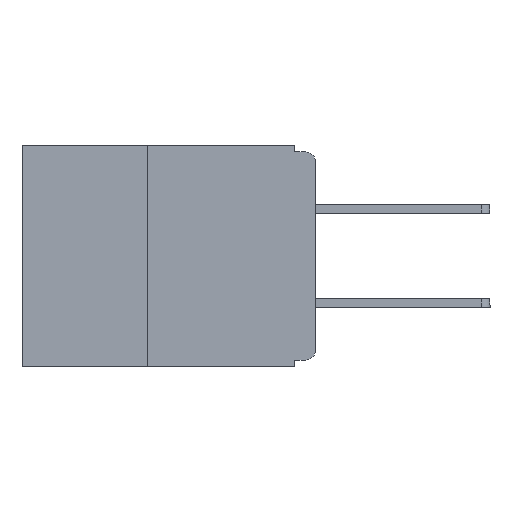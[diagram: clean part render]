
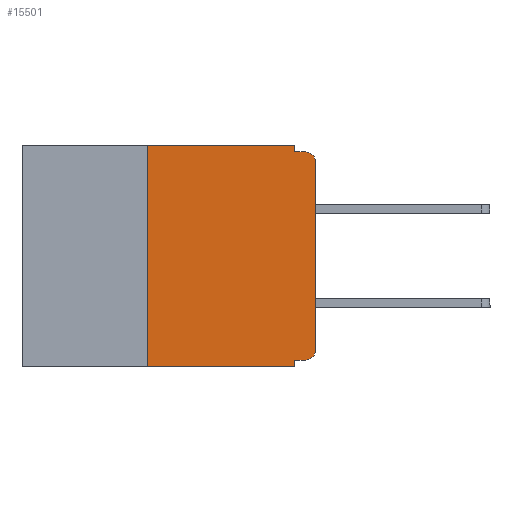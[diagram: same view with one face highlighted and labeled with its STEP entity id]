
A CAD part, left-side view. The second image highlights one B-rep face of the part: STEP entity #15501.
In plain terms, the highlighted planar face has unit normal (-1, 0, 0).
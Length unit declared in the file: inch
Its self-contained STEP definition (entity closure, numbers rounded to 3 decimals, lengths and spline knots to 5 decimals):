
#93 = DIRECTION ( 'NONE',  ( 0., 0., 1. ) ) ;
#161 = DIRECTION ( 'NONE',  ( 0., 0., -1. ) ) ;
#200 = EDGE_CURVE ( 'NONE', #10497, #10987, #3609, .T. ) ;
#527 = ORIENTED_EDGE ( 'NONE', *, *, #200, .T. ) ;
#879 = CARTESIAN_POINT ( 'NONE',  ( 0., 0., -0.025 ) ) ;
#891 = EDGE_CURVE ( 'NONE', #6272, #3194, #23854, .T. ) ;
#1140 = VECTOR ( 'NONE', #13834, 39.37008 ) ;
#1206 = CARTESIAN_POINT ( 'NONE',  ( 0., 0., -0.305 ) ) ;
#1431 = VECTOR ( 'NONE', #21954, 39.37008 ) ;
#2055 = LINE ( 'NONE', #20069, #1431 ) ;
#2853 = VECTOR ( 'NONE', #23637, 39.37008 ) ;
#2869 = EDGE_CURVE ( 'NONE', #10497, #3368, #5034, .T. ) ;
#3194 = VERTEX_POINT ( 'NONE', #1206 ) ;
#3368 = VERTEX_POINT ( 'NONE', #19367 ) ;
#3384 = CARTESIAN_POINT ( 'NONE',  ( 0., 0.437, 0. ) ) ;
#3609 = LINE ( 'NONE', #6363, #23599 ) ;
#3759 = CARTESIAN_POINT ( 'NONE',  ( 0., 0.015, -0.305 ) ) ;
#3777 = VECTOR ( 'NONE', #93, 39.37008 ) ;
#3789 = LINE ( 'NONE', #12873, #18228 ) ;
#4226 = EDGE_CURVE ( 'NONE', #16922, #5382, #19098, .T. ) ;
#4270 = ORIENTED_EDGE ( 'NONE', *, *, #4414, .T. ) ;
#4317 = CARTESIAN_POINT ( 'NONE',  ( 0., 0.015, -0.025 ) ) ;
#4382 = VERTEX_POINT ( 'NONE', #879 ) ;
#4414 = EDGE_CURVE ( 'NONE', #3194, #4382, #3789, .T. ) ;
#5034 = LINE ( 'NONE', #8023, #3777 ) ;
#5382 = VERTEX_POINT ( 'NONE', #17486 ) ;
#5412 = DIRECTION ( 'NONE',  ( 0., -1., 0. ) ) ;
#5519 = ORIENTED_EDGE ( 'NONE', *, *, #19299, .F. ) ;
#5789 = VERTEX_POINT ( 'NONE', #6848 ) ;
#5913 = CARTESIAN_POINT ( 'NONE',  ( 0., 0.031, -0.33 ) ) ;
#6272 = VERTEX_POINT ( 'NONE', #6315 ) ;
#6315 = CARTESIAN_POINT ( 'NONE',  ( 0., 0.015, -0.32 ) ) ;
#6341 = DIRECTION ( 'NONE',  ( 0., 0., -1. ) ) ;
#6363 = CARTESIAN_POINT ( 'NONE',  ( 0., 0.437, -0.33 ) ) ;
#6452 = LINE ( 'NONE', #5913, #1140 ) ;
#6473 = ORIENTED_EDGE ( 'NONE', *, *, #19109, .F. ) ;
#6848 = CARTESIAN_POINT ( 'NONE',  ( 0., 0.031, -0.32 ) ) ;
#7182 = CARTESIAN_POINT ( 'NONE',  ( 0., 0., -0.32 ) ) ;
#7573 = EDGE_CURVE ( 'NONE', #4382, #18886, #15102, .T. ) ;
#7706 = ORIENTED_EDGE ( 'NONE', *, *, #891, .T. ) ;
#7726 = AXIS2_PLACEMENT_3D ( 'NONE', #15925, #12072, #161 ) ;
#7989 = DIRECTION ( 'NONE',  ( 0., -1., 0. ) ) ;
#8023 = CARTESIAN_POINT ( 'NONE',  ( 0., 0.25, -0.33 ) ) ;
#10107 = PLANE ( 'NONE',  #7726 ) ;
#10197 = ORIENTED_EDGE ( 'NONE', *, *, #7573, .T. ) ;
#10256 = EDGE_CURVE ( 'NONE', #6272, #5789, #22152, .T. ) ;
#10322 = CARTESIAN_POINT ( 'NONE',  ( 0., 0.031, 0. ) ) ;
#10497 = VERTEX_POINT ( 'NONE', #11944 ) ;
#10820 = AXIS2_PLACEMENT_3D ( 'NONE', #3759, #22332, #20162 ) ;
#10915 = DIRECTION ( 'NONE',  ( 0., 0., 1. ) ) ;
#10987 = VERTEX_POINT ( 'NONE', #17690 ) ;
#11100 = DIRECTION ( 'NONE',  ( 0., 1., 0. ) ) ;
#11944 = CARTESIAN_POINT ( 'NONE',  ( 0., 0.25, -0.33 ) ) ;
#12041 = ORIENTED_EDGE ( 'NONE', *, *, #17870, .F. ) ;
#12072 = DIRECTION ( 'NONE',  ( 1., 0., 0. ) ) ;
#12873 = CARTESIAN_POINT ( 'NONE',  ( 0., 0., 0. ) ) ;
#13834 = DIRECTION ( 'NONE',  ( 0., 0., -1. ) ) ;
#15102 = CIRCLE ( 'NONE', #15833, 0.015 ) ;
#15501 = ADVANCED_FACE ( 'NONE', ( #20167 ), #10107, .F. ) ;
#15714 = EDGE_LOOP ( 'NONE', ( #4270, #10197, #5519, #16607, #12041, #24472, #527, #6473, #16913, #7706 ) ) ;
#15833 = AXIS2_PLACEMENT_3D ( 'NONE', #4317, #18046, #6341 ) ;
#15925 = CARTESIAN_POINT ( 'NONE',  ( 0., 0.437, 0. ) ) ;
#16607 = ORIENTED_EDGE ( 'NONE', *, *, #4226, .F. ) ;
#16913 = ORIENTED_EDGE ( 'NONE', *, *, #10256, .F. ) ;
#16922 = VERTEX_POINT ( 'NONE', #22348 ) ;
#16960 = VECTOR ( 'NONE', #5412, 39.37008 ) ;
#17486 = CARTESIAN_POINT ( 'NONE',  ( 0., 0.031, -0.01 ) ) ;
#17690 = CARTESIAN_POINT ( 'NONE',  ( 0., 0.031, -0.33 ) ) ;
#17870 = EDGE_CURVE ( 'NONE', #3368, #16922, #21942, .T. ) ;
#18046 = DIRECTION ( 'NONE',  ( -1., 0., 0. ) ) ;
#18228 = VECTOR ( 'NONE', #10915, 39.37008 ) ;
#18862 = CARTESIAN_POINT ( 'NONE',  ( 0., 0.015, -0.01 ) ) ;
#18886 = VERTEX_POINT ( 'NONE', #18862 ) ;
#19098 = LINE ( 'NONE', #10322, #2853 ) ;
#19109 = EDGE_CURVE ( 'NONE', #5789, #10987, #6452, .T. ) ;
#19299 = EDGE_CURVE ( 'NONE', #5382, #18886, #2055, .T. ) ;
#19367 = CARTESIAN_POINT ( 'NONE',  ( 0., 0.25, 0. ) ) ;
#20069 = CARTESIAN_POINT ( 'NONE',  ( 0., 0., -0.01 ) ) ;
#20162 = DIRECTION ( 'NONE',  ( 0., 0., -1. ) ) ;
#20167 = FACE_OUTER_BOUND ( 'NONE', #15714, .T. ) ;
#21580 = VECTOR ( 'NONE', #11100, 39.37008 ) ;
#21942 = LINE ( 'NONE', #3384, #16960 ) ;
#21954 = DIRECTION ( 'NONE',  ( 0., -1., 0. ) ) ;
#22152 = LINE ( 'NONE', #7182, #21580 ) ;
#22332 = DIRECTION ( 'NONE',  ( -1., 0., 0. ) ) ;
#22348 = CARTESIAN_POINT ( 'NONE',  ( 0., 0.031, 0. ) ) ;
#23599 = VECTOR ( 'NONE', #7989, 39.37008 ) ;
#23637 = DIRECTION ( 'NONE',  ( 0., 0., -1. ) ) ;
#23854 = CIRCLE ( 'NONE', #10820, 0.015 ) ;
#24472 = ORIENTED_EDGE ( 'NONE', *, *, #2869, .F. ) ;
